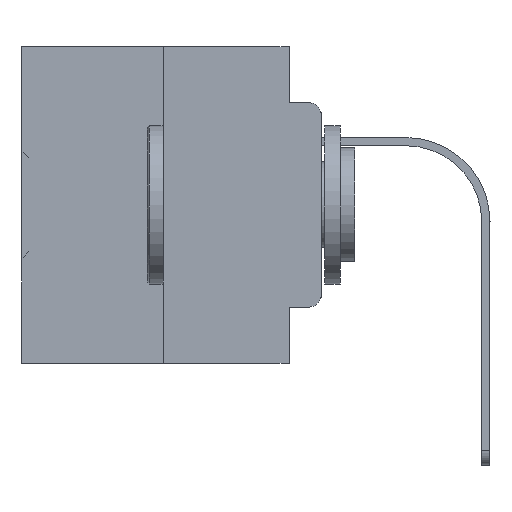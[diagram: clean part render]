
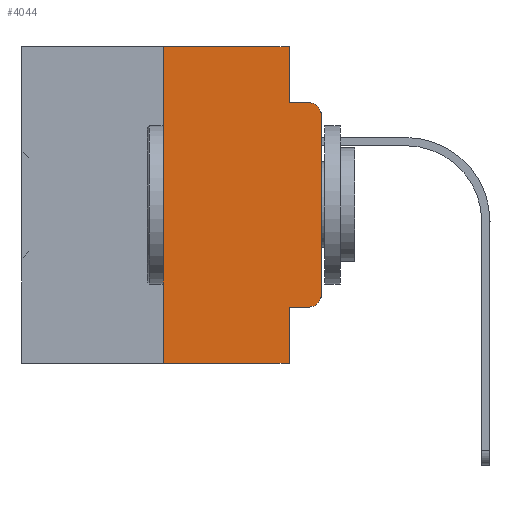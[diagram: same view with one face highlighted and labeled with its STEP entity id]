
A CAD part, left-side view. The second image highlights one B-rep face of the part: STEP entity #4044.
In plain terms, the highlighted planar face has unit normal (-1, 0, 0).
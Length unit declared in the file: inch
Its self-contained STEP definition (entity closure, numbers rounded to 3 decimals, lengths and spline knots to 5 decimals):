
#524 = LINE ( 'NONE', #24228, #23422 ) ;
#1189 = CARTESIAN_POINT ( 'NONE',  ( 0., 0.02, -0.0885 ) ) ;
#1417 = CARTESIAN_POINT ( 'NONE',  ( 0., 0., 0. ) ) ;
#1524 = VECTOR ( 'NONE', #37039, 39.37008 ) ;
#2923 = DIRECTION ( 'NONE',  ( 0., 0., 1. ) ) ;
#3903 = CARTESIAN_POINT ( 'NONE',  ( 0., 0.473, 0. ) ) ;
#3988 = ORIENTED_EDGE ( 'NONE', *, *, #23157, .T. ) ;
#4044 = ADVANCED_FACE ( 'NONE', ( #36121 ), #27731, .F. ) ;
#4133 = VERTEX_POINT ( 'NONE', #12948 ) ;
#4800 = ORIENTED_EDGE ( 'NONE', *, *, #20721, .F. ) ;
#5772 = AXIS2_PLACEMENT_3D ( 'NONE', #23851, #17589, #5853 ) ;
#5853 = DIRECTION ( 'NONE',  ( 0., 0., -1. ) ) ;
#6295 = AXIS2_PLACEMENT_3D ( 'NONE', #18580, #30491, #19940 ) ;
#6440 = CARTESIAN_POINT ( 'NONE',  ( 0., 0.473, 0. ) ) ;
#9349 = EDGE_CURVE ( 'NONE', #28681, #4133, #25709, .T. ) ;
#9475 = VECTOR ( 'NONE', #16904, 39.37008 ) ;
#10223 = DIRECTION ( 'NONE',  ( 0., 0., 1. ) ) ;
#10275 = ORIENTED_EDGE ( 'NONE', *, *, #9349, .F. ) ;
#11116 = EDGE_CURVE ( 'NONE', #20741, #4133, #19842, .T. ) ;
#11367 = DIRECTION ( 'NONE',  ( 0., -1., 0. ) ) ;
#11481 = ORIENTED_EDGE ( 'NONE', *, *, #15540, .T. ) ;
#12241 = LINE ( 'NONE', #1417, #36949 ) ;
#12278 = VECTOR ( 'NONE', #22601, 39.37008 ) ;
#12709 = LINE ( 'NONE', #3903, #32074 ) ;
#12923 = ORIENTED_EDGE ( 'NONE', *, *, #35273, .T. ) ;
#12948 = CARTESIAN_POINT ( 'NONE',  ( 0., 0.051, -0.5 ) ) ;
#13124 = ORIENTED_EDGE ( 'NONE', *, *, #11116, .T. ) ;
#13364 = AXIS2_PLACEMENT_3D ( 'NONE', #6440, #24048, #18363 ) ;
#13538 = CARTESIAN_POINT ( 'NONE',  ( 0., 0.051, -0.0885 ) ) ;
#13581 = CARTESIAN_POINT ( 'NONE',  ( 0., 0.473, -0.5 ) ) ;
#13866 = VERTEX_POINT ( 'NONE', #1189 ) ;
#13897 = CARTESIAN_POINT ( 'NONE',  ( 0., 0., -0.3915 ) ) ;
#14304 = CARTESIAN_POINT ( 'NONE',  ( 0., 0.25, 0. ) ) ;
#15540 = EDGE_CURVE ( 'NONE', #17970, #13866, #17547, .T. ) ;
#16397 = CARTESIAN_POINT ( 'NONE',  ( 0., 0.02, -0.4115 ) ) ;
#16733 = CARTESIAN_POINT ( 'NONE',  ( 0., 0.051, 0. ) ) ;
#16904 = DIRECTION ( 'NONE',  ( 0., 0., -1. ) ) ;
#16927 = LINE ( 'NONE', #34114, #1524 ) ;
#17547 = CIRCLE ( 'NONE', #6295, 0.02 ) ;
#17589 = DIRECTION ( 'NONE',  ( -1., 0., 0. ) ) ;
#17970 = VERTEX_POINT ( 'NONE', #35005 ) ;
#18363 = DIRECTION ( 'NONE',  ( 0., 0., -1. ) ) ;
#18580 = CARTESIAN_POINT ( 'NONE',  ( 0., 0.02, -0.1085 ) ) ;
#18813 = ORIENTED_EDGE ( 'NONE', *, *, #24804, .F. ) ;
#19688 = VERTEX_POINT ( 'NONE', #34585 ) ;
#19842 = LINE ( 'NONE', #13581, #12278 ) ;
#19940 = DIRECTION ( 'NONE',  ( 0., 0., -1. ) ) ;
#20363 = CARTESIAN_POINT ( 'NONE',  ( 0., 0.25, -0.5 ) ) ;
#20721 = EDGE_CURVE ( 'NONE', #32875, #13866, #34638, .T. ) ;
#20741 = VERTEX_POINT ( 'NONE', #20363 ) ;
#21682 = ORIENTED_EDGE ( 'NONE', *, *, #31974, .F. ) ;
#22601 = DIRECTION ( 'NONE',  ( 0., -1., 0. ) ) ;
#23157 = EDGE_CURVE ( 'NONE', #26207, #17970, #12241, .T. ) ;
#23422 = VECTOR ( 'NONE', #35747, 39.37008 ) ;
#23492 = LINE ( 'NONE', #14304, #34371 ) ;
#23851 = CARTESIAN_POINT ( 'NONE',  ( 0., 0.02, -0.3915 ) ) ;
#24048 = DIRECTION ( 'NONE',  ( 1., 0., 0. ) ) ;
#24228 = CARTESIAN_POINT ( 'NONE',  ( 0., 0.051, -0.4115 ) ) ;
#24804 = EDGE_CURVE ( 'NONE', #19688, #28203, #12709, .T. ) ;
#24933 = CARTESIAN_POINT ( 'NONE',  ( 0., 0.051, -0.0885 ) ) ;
#25354 = VERTEX_POINT ( 'NONE', #16397 ) ;
#25668 = EDGE_CURVE ( 'NONE', #28203, #32875, #16927, .T. ) ;
#25709 = LINE ( 'NONE', #34679, #9475 ) ;
#26207 = VERTEX_POINT ( 'NONE', #13897 ) ;
#26303 = VECTOR ( 'NONE', #11367, 39.37008 ) ;
#26325 = EDGE_LOOP ( 'NONE', ( #3988, #11481, #4800, #27091, #18813, #21682, #13124, #10275, #35337, #12923 ) ) ;
#27091 = ORIENTED_EDGE ( 'NONE', *, *, #25668, .F. ) ;
#27731 = PLANE ( 'NONE',  #13364 ) ;
#28171 = DIRECTION ( 'NONE',  ( 0., -1., 0. ) ) ;
#28203 = VERTEX_POINT ( 'NONE', #16733 ) ;
#28681 = VERTEX_POINT ( 'NONE', #30567 ) ;
#30491 = DIRECTION ( 'NONE',  ( -1., 0., 0. ) ) ;
#30567 = CARTESIAN_POINT ( 'NONE',  ( 0., 0.051, -0.4115 ) ) ;
#31974 = EDGE_CURVE ( 'NONE', #20741, #19688, #23492, .T. ) ;
#32074 = VECTOR ( 'NONE', #28171, 39.37008 ) ;
#32875 = VERTEX_POINT ( 'NONE', #24933 ) ;
#34114 = CARTESIAN_POINT ( 'NONE',  ( 0., 0.051, 0. ) ) ;
#34371 = VECTOR ( 'NONE', #2923, 39.37008 ) ;
#34585 = CARTESIAN_POINT ( 'NONE',  ( 0., 0.25, 0. ) ) ;
#34638 = LINE ( 'NONE', #13538, #26303 ) ;
#34679 = CARTESIAN_POINT ( 'NONE',  ( 0., 0.051, 0. ) ) ;
#35005 = CARTESIAN_POINT ( 'NONE',  ( 0., 0., -0.1085 ) ) ;
#35273 = EDGE_CURVE ( 'NONE', #25354, #26207, #37598, .T. ) ;
#35337 = ORIENTED_EDGE ( 'NONE', *, *, #38225, .T. ) ;
#35747 = DIRECTION ( 'NONE',  ( 0., -1., 0. ) ) ;
#36121 = FACE_OUTER_BOUND ( 'NONE', #26325, .T. ) ;
#36949 = VECTOR ( 'NONE', #10223, 39.37008 ) ;
#37039 = DIRECTION ( 'NONE',  ( 0., 0., -1. ) ) ;
#37598 = CIRCLE ( 'NONE', #5772, 0.02 ) ;
#38225 = EDGE_CURVE ( 'NONE', #28681, #25354, #524, .T. ) ;
